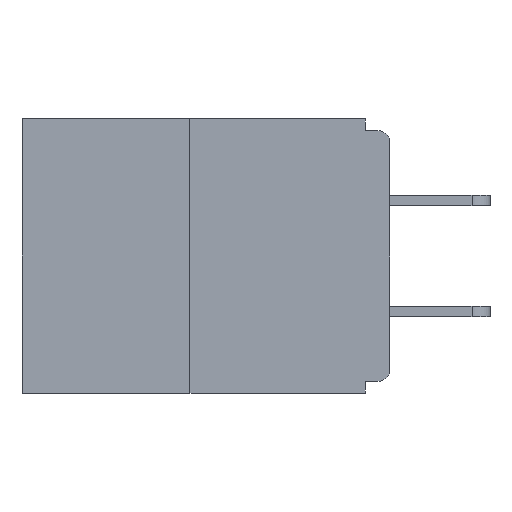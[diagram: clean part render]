
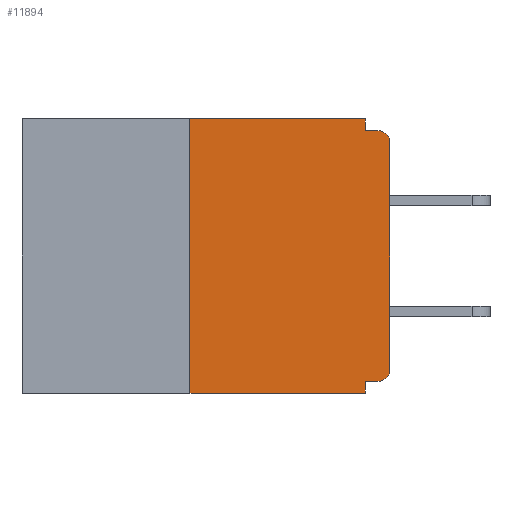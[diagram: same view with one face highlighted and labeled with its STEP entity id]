
A CAD part, left-side view. The second image highlights one B-rep face of the part: STEP entity #11894.
In plain terms, the highlighted planar face has unit normal (-1, 0, 0).
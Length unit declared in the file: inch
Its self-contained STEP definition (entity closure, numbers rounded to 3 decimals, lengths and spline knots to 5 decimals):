
#423 = FACE_OUTER_BOUND ( 'NONE', #4611, .T. ) ;
#564 = CARTESIAN_POINT ( 'NONE',  ( 0., 0., -0.03 ) ) ;
#739 = VECTOR ( 'NONE', #12146, 39.37008 ) ;
#746 = CARTESIAN_POINT ( 'NONE',  ( 0., 0.015, -0.03 ) ) ;
#1517 = EDGE_CURVE ( 'NONE', #7093, #15506, #18446, .T. ) ;
#2293 = CARTESIAN_POINT ( 'NONE',  ( 0., 0.031, 0. ) ) ;
#3446 = VECTOR ( 'NONE', #8028, 39.37008 ) ;
#3504 = VERTEX_POINT ( 'NONE', #4042 ) ;
#3530 = EDGE_CURVE ( 'NONE', #3504, #20780, #7103, .T. ) ;
#3593 = DIRECTION ( 'NONE',  ( 0., 1., 0. ) ) ;
#3609 = EDGE_CURVE ( 'NONE', #15335, #20837, #5496, .T. ) ;
#4042 = CARTESIAN_POINT ( 'NONE',  ( 0., 0.25, -0.343 ) ) ;
#4325 = CARTESIAN_POINT ( 'NONE',  ( 0., 0.031, -0.328 ) ) ;
#4611 = EDGE_LOOP ( 'NONE', ( #18285, #21702, #15214, #18568, #16358, #17914, #10872, #6890, #7681, #16955 ) ) ;
#5496 = LINE ( 'NONE', #6774, #10926 ) ;
#5515 = CARTESIAN_POINT ( 'NONE',  ( 0., 0.015, -0.015 ) ) ;
#5979 = VERTEX_POINT ( 'NONE', #14060 ) ;
#6068 = CARTESIAN_POINT ( 'NONE',  ( 0., 0.25, 0. ) ) ;
#6764 = DIRECTION ( 'NONE',  ( 0., 0., -1. ) ) ;
#6774 = CARTESIAN_POINT ( 'NONE',  ( 0., 0., 0. ) ) ;
#6890 = ORIENTED_EDGE ( 'NONE', *, *, #25226, .T. ) ;
#7093 = VERTEX_POINT ( 'NONE', #17504 ) ;
#7103 = LINE ( 'NONE', #6068, #739 ) ;
#7681 = ORIENTED_EDGE ( 'NONE', *, *, #1517, .F. ) ;
#7971 = AXIS2_PLACEMENT_3D ( 'NONE', #21643, #19604, #21819 ) ;
#8028 = DIRECTION ( 'NONE',  ( 0., 0., -1. ) ) ;
#8240 = EDGE_CURVE ( 'NONE', #5979, #25572, #14912, .T. ) ;
#8653 = EDGE_CURVE ( 'NONE', #5979, #15335, #16170, .T. ) ;
#8790 = VECTOR ( 'NONE', #3593, 39.37008 ) ;
#9045 = VERTEX_POINT ( 'NONE', #18553 ) ;
#9486 = LINE ( 'NONE', #26236, #3446 ) ;
#9634 = CARTESIAN_POINT ( 'NONE',  ( 0., 0., -0.328 ) ) ;
#9742 = EDGE_CURVE ( 'NONE', #25572, #9045, #9486, .T. ) ;
#10389 = VECTOR ( 'NONE', #13564, 39.37008 ) ;
#10663 = AXIS2_PLACEMENT_3D ( 'NONE', #746, #10829, #14803 ) ;
#10829 = DIRECTION ( 'NONE',  ( -1., 0., 0. ) ) ;
#10838 = CARTESIAN_POINT ( 'NONE',  ( 0., 0.46, -0.343 ) ) ;
#10872 = ORIENTED_EDGE ( 'NONE', *, *, #3609, .T. ) ;
#10926 = VECTOR ( 'NONE', #24990, 39.37008 ) ;
#11894 = ADVANCED_FACE ( 'NONE', ( #423 ), #25719, .F. ) ;
#12080 = CARTESIAN_POINT ( 'NONE',  ( 0., 0.46, 0. ) ) ;
#12146 = DIRECTION ( 'NONE',  ( 0., 0., 1. ) ) ;
#12677 = EDGE_CURVE ( 'NONE', #20491, #7093, #12841, .T. ) ;
#12841 = LINE ( 'NONE', #13215, #23454 ) ;
#13215 = CARTESIAN_POINT ( 'NONE',  ( 0., 0.031, 0. ) ) ;
#13270 = CARTESIAN_POINT ( 'NONE',  ( 0., 0.25, 0. ) ) ;
#13564 = DIRECTION ( 'NONE',  ( 0., -1., 0. ) ) ;
#14060 = CARTESIAN_POINT ( 'NONE',  ( 0., 0.015, -0.328 ) ) ;
#14803 = DIRECTION ( 'NONE',  ( 0., 0., -1. ) ) ;
#14912 = LINE ( 'NONE', #9634, #8790 ) ;
#15214 = ORIENTED_EDGE ( 'NONE', *, *, #17389, .T. ) ;
#15335 = VERTEX_POINT ( 'NONE', #20847 ) ;
#15506 = VERTEX_POINT ( 'NONE', #5515 ) ;
#16170 = CIRCLE ( 'NONE', #23699, 0.015 ) ;
#16358 = ORIENTED_EDGE ( 'NONE', *, *, #8240, .F. ) ;
#16434 = EDGE_CURVE ( 'NONE', #20780, #20491, #24014, .T. ) ;
#16955 = ORIENTED_EDGE ( 'NONE', *, *, #12677, .F. ) ;
#17134 = DIRECTION ( 'NONE',  ( 0., -1., 0. ) ) ;
#17389 = EDGE_CURVE ( 'NONE', #3504, #9045, #20747, .T. ) ;
#17504 = CARTESIAN_POINT ( 'NONE',  ( 0., 0.031, -0.015 ) ) ;
#17914 = ORIENTED_EDGE ( 'NONE', *, *, #8653, .T. ) ;
#18285 = ORIENTED_EDGE ( 'NONE', *, *, #16434, .F. ) ;
#18446 = LINE ( 'NONE', #19492, #10389 ) ;
#18553 = CARTESIAN_POINT ( 'NONE',  ( 0., 0.031, -0.343 ) ) ;
#18568 = ORIENTED_EDGE ( 'NONE', *, *, #9742, .F. ) ;
#18574 = VECTOR ( 'NONE', #26558, 39.37008 ) ;
#19059 = DIRECTION ( 'NONE',  ( -1., 0., 0. ) ) ;
#19459 = VECTOR ( 'NONE', #17134, 39.37008 ) ;
#19492 = CARTESIAN_POINT ( 'NONE',  ( 0., 0., -0.015 ) ) ;
#19604 = DIRECTION ( 'NONE',  ( 1., 0., 0. ) ) ;
#19912 = CIRCLE ( 'NONE', #10663, 0.015 ) ;
#20491 = VERTEX_POINT ( 'NONE', #2293 ) ;
#20747 = LINE ( 'NONE', #10838, #19459 ) ;
#20780 = VERTEX_POINT ( 'NONE', #13270 ) ;
#20837 = VERTEX_POINT ( 'NONE', #564 ) ;
#20847 = CARTESIAN_POINT ( 'NONE',  ( 0., 0., -0.313 ) ) ;
#20999 = CARTESIAN_POINT ( 'NONE',  ( 0., 0.015, -0.313 ) ) ;
#21365 = DIRECTION ( 'NONE',  ( 0., 0., -1. ) ) ;
#21643 = CARTESIAN_POINT ( 'NONE',  ( 0., 0.46, 0. ) ) ;
#21702 = ORIENTED_EDGE ( 'NONE', *, *, #3530, .F. ) ;
#21819 = DIRECTION ( 'NONE',  ( 0., 0., -1. ) ) ;
#23454 = VECTOR ( 'NONE', #21365, 39.37008 ) ;
#23699 = AXIS2_PLACEMENT_3D ( 'NONE', #20999, #19059, #6764 ) ;
#24014 = LINE ( 'NONE', #12080, #18574 ) ;
#24990 = DIRECTION ( 'NONE',  ( 0., 0., 1. ) ) ;
#25226 = EDGE_CURVE ( 'NONE', #20837, #15506, #19912, .T. ) ;
#25572 = VERTEX_POINT ( 'NONE', #4325 ) ;
#25719 = PLANE ( 'NONE',  #7971 ) ;
#26236 = CARTESIAN_POINT ( 'NONE',  ( 0., 0.031, -0.343 ) ) ;
#26558 = DIRECTION ( 'NONE',  ( 0., -1., 0. ) ) ;
